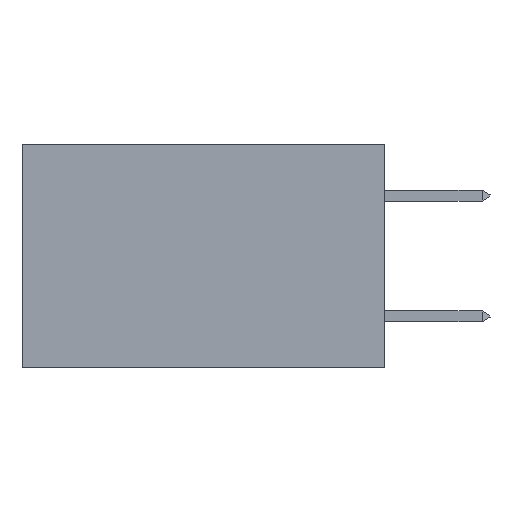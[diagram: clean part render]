
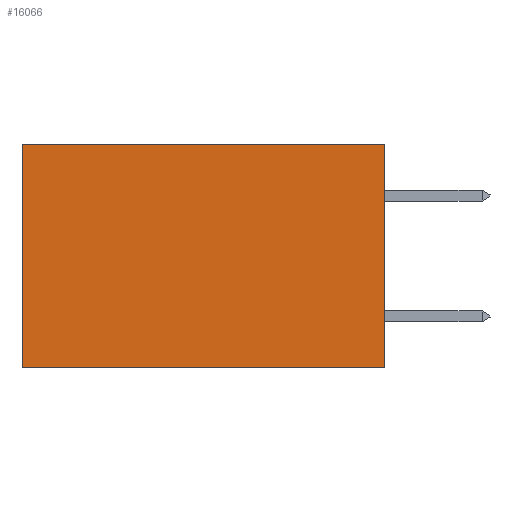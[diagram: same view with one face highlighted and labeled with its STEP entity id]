
A CAD part, left-side view. The second image highlights one B-rep face of the part: STEP entity #16066.
In plain terms, the highlighted planar face has unit normal (-1, 0, 0).
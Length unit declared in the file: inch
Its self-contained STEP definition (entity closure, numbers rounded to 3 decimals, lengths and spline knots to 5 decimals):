
#4130 = DIRECTION ( 'NONE',  ( 0., 0., -1. ) ) ;
#4802 = VECTOR ( 'NONE', #38441, 39.37008 ) ;
#5221 = EDGE_CURVE ( 'NONE', #37312, #35661, #11393, .T. ) ;
#5379 = VECTOR ( 'NONE', #43208, 39.37008 ) ;
#8313 = EDGE_LOOP ( 'NONE', ( #29644, #22275, #39979, #12513 ) ) ;
#9601 = AXIS2_PLACEMENT_3D ( 'NONE', #10513, #27923, #14368 ) ;
#10125 = DIRECTION ( 'NONE',  ( 0., 1., 0. ) ) ;
#10513 = CARTESIAN_POINT ( 'NONE',  ( 0.2875, 0., 0. ) ) ;
#10768 = CARTESIAN_POINT ( 'NONE',  ( 0.2875, 0.6, 0. ) ) ;
#11031 = CARTESIAN_POINT ( 'NONE',  ( 0.2875, 0.6, 0. ) ) ;
#11393 = LINE ( 'NONE', #40405, #16700 ) ;
#11766 = CARTESIAN_POINT ( 'NONE',  ( 0.2875, 0., -0.37 ) ) ;
#12513 = ORIENTED_EDGE ( 'NONE', *, *, #5221, .T. ) ;
#14368 = DIRECTION ( 'NONE',  ( 0., 0., -1. ) ) ;
#14766 = EDGE_CURVE ( 'NONE', #38260, #27584, #40930, .T. ) ;
#16055 = CARTESIAN_POINT ( 'NONE',  ( 0.2875, 0., -0.37 ) ) ;
#16066 = ADVANCED_FACE ( 'NONE', ( #23899 ), #17464, .F. ) ;
#16218 = EDGE_CURVE ( 'NONE', #37312, #38260, #33987, .T. ) ;
#16700 = VECTOR ( 'NONE', #10125, 39.37008 ) ;
#17464 = PLANE ( 'NONE',  #9601 ) ;
#22275 = ORIENTED_EDGE ( 'NONE', *, *, #14766, .F. ) ;
#23899 = FACE_OUTER_BOUND ( 'NONE', #8313, .T. ) ;
#25326 = LINE ( 'NONE', #10768, #32767 ) ;
#27584 = VERTEX_POINT ( 'NONE', #40420 ) ;
#27923 = DIRECTION ( 'NONE',  ( 1., 0., 0. ) ) ;
#29644 = ORIENTED_EDGE ( 'NONE', *, *, #43061, .T. ) ;
#32767 = VECTOR ( 'NONE', #4130, 39.37008 ) ;
#33987 = LINE ( 'NONE', #35473, #4802 ) ;
#35473 = CARTESIAN_POINT ( 'NONE',  ( 0.2875, 0., 0. ) ) ;
#35661 = VERTEX_POINT ( 'NONE', #11031 ) ;
#37312 = VERTEX_POINT ( 'NONE', #40297 ) ;
#38260 = VERTEX_POINT ( 'NONE', #11766 ) ;
#38441 = DIRECTION ( 'NONE',  ( 0., 0., -1. ) ) ;
#39979 = ORIENTED_EDGE ( 'NONE', *, *, #16218, .F. ) ;
#40297 = CARTESIAN_POINT ( 'NONE',  ( 0.2875, 0., 0. ) ) ;
#40405 = CARTESIAN_POINT ( 'NONE',  ( 0.2875, 0., 0. ) ) ;
#40420 = CARTESIAN_POINT ( 'NONE',  ( 0.2875, 0.6, -0.37 ) ) ;
#40930 = LINE ( 'NONE', #16055, #5379 ) ;
#43061 = EDGE_CURVE ( 'NONE', #35661, #27584, #25326, .T. ) ;
#43208 = DIRECTION ( 'NONE',  ( 0., 1., 0. ) ) ;
